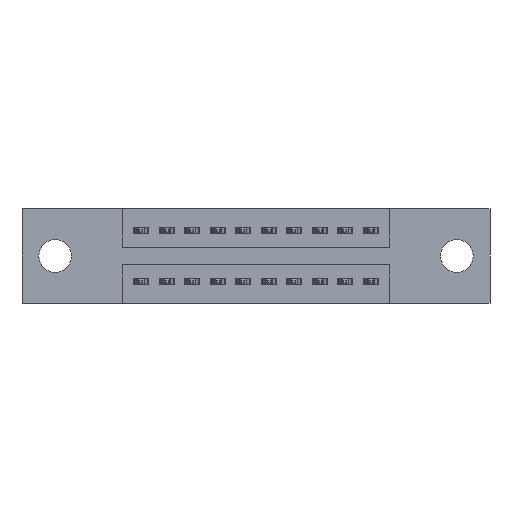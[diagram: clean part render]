
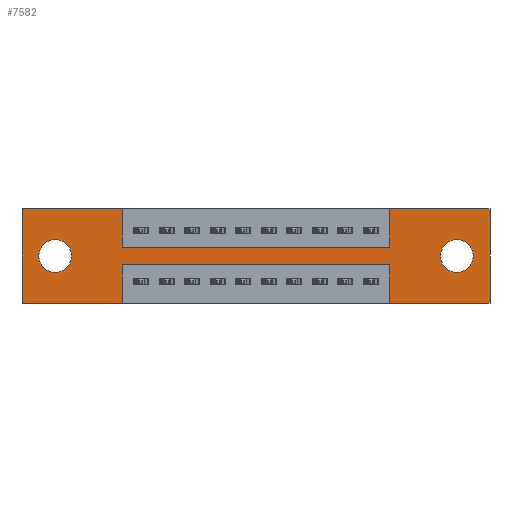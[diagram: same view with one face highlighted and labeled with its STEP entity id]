
A CAD part, front view. The second image highlights one B-rep face of the part: STEP entity #7582.
In plain terms, the highlighted planar face has unit normal (0, -1, 0).
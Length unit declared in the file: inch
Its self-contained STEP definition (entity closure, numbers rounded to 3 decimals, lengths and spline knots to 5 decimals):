
#117 = ORIENTED_EDGE ( 'NONE', *, *, #8578, .T. ) ;
#363 = DIRECTION ( 'NONE',  ( 0., 0., 1. ) ) ;
#426 = EDGE_CURVE ( 'NONE', #10131, #4651, #6226, .T. ) ;
#573 = CIRCLE ( 'NONE', #4026, 0.064 ) ;
#599 = EDGE_CURVE ( 'NONE', #11635, #8433, #9215, .T. ) ;
#674 = DIRECTION ( 'NONE',  ( 0., 1., 0. ) ) ;
#698 = ORIENTED_EDGE ( 'NONE', *, *, #4760, .T. ) ;
#797 = VERTEX_POINT ( 'NONE', #4921 ) ;
#798 = DIRECTION ( 'NONE',  ( 0., 1., 0. ) ) ;
#901 = CARTESIAN_POINT ( 'NONE',  ( 1.4425, 0., -0.15 ) ) ;
#910 = DIRECTION ( 'NONE',  ( -1., 0., 0. ) ) ;
#1157 = ORIENTED_EDGE ( 'NONE', *, *, #7552, .F. ) ;
#1232 = CARTESIAN_POINT ( 'NONE',  ( 1.705, 0., -0.185 ) ) ;
#1618 = CARTESIAN_POINT ( 'NONE',  ( 0.13, 0., -0.185 ) ) ;
#1696 = LINE ( 'NONE', #4581, #8347 ) ;
#1740 = CARTESIAN_POINT ( 'NONE',  ( 0.13, 0., -0.121 ) ) ;
#1905 = VERTEX_POINT ( 'NONE', #1740 ) ;
#2096 = LINE ( 'NONE', #7537, #6650 ) ;
#2200 = DIRECTION ( 'NONE',  ( 0., 1., 0. ) ) ;
#2248 = VECTOR ( 'NONE', #10464, 39.37008 ) ;
#2322 = CIRCLE ( 'NONE', #6504, 0.064 ) ;
#2341 = DIRECTION ( 'NONE',  ( 0., -1., 0. ) ) ;
#2364 = CARTESIAN_POINT ( 'NONE',  ( 1.4425, 0., 0. ) ) ;
#2391 = VECTOR ( 'NONE', #3422, 39.37008 ) ;
#2468 = VECTOR ( 'NONE', #910, 39.37008 ) ;
#2492 = CARTESIAN_POINT ( 'NONE',  ( 0., 0., 0. ) ) ;
#2693 = VECTOR ( 'NONE', #5225, 39.37008 ) ;
#2758 = CARTESIAN_POINT ( 'NONE',  ( 1.835, 0., 0. ) ) ;
#2976 = CARTESIAN_POINT ( 'NONE',  ( 0., 0., 0. ) ) ;
#2991 = CIRCLE ( 'NONE', #7882, 0.064 ) ;
#3112 = EDGE_CURVE ( 'NONE', #9132, #5000, #3172, .T. ) ;
#3153 = LINE ( 'NONE', #5531, #10993 ) ;
#3172 = LINE ( 'NONE', #9256, #10413 ) ;
#3190 = VERTEX_POINT ( 'NONE', #10410 ) ;
#3262 = CARTESIAN_POINT ( 'NONE',  ( 1.705, 0., -0.249 ) ) ;
#3422 = DIRECTION ( 'NONE',  ( 1., 0., 0. ) ) ;
#3828 = CARTESIAN_POINT ( 'NONE',  ( 1.4425, 0., -0.37 ) ) ;
#3977 = DIRECTION ( 'NONE',  ( 0., 0., -1. ) ) ;
#4008 = EDGE_LOOP ( 'NONE', ( #9153, #8576, #11238, #9944, #4397, #11677, #10538, #4881, #1157, #10408, #7628, #12001 ) ) ;
#4026 = AXIS2_PLACEMENT_3D ( 'NONE', #1618, #674, #10848 ) ;
#4397 = ORIENTED_EDGE ( 'NONE', *, *, #9378, .F. ) ;
#4581 = CARTESIAN_POINT ( 'NONE',  ( 0., 0., 0. ) ) ;
#4601 = CARTESIAN_POINT ( 'NONE',  ( 0., 0., -0.37 ) ) ;
#4606 = EDGE_CURVE ( 'NONE', #4651, #7779, #1696, .T. ) ;
#4651 = VERTEX_POINT ( 'NONE', #7466 ) ;
#4669 = EDGE_LOOP ( 'NONE', ( #698, #10073 ) ) ;
#4760 = EDGE_CURVE ( 'NONE', #797, #10524, #2991, .T. ) ;
#4812 = CARTESIAN_POINT ( 'NONE',  ( 0.3925, 0., 0. ) ) ;
#4881 = ORIENTED_EDGE ( 'NONE', *, *, #11899, .F. ) ;
#4921 = CARTESIAN_POINT ( 'NONE',  ( 1.705, 0., -0.121 ) ) ;
#5000 = VERTEX_POINT ( 'NONE', #2976 ) ;
#5011 = DIRECTION ( 'NONE',  ( 0., 1., 0. ) ) ;
#5141 = CARTESIAN_POINT ( 'NONE',  ( 0.13, 0., -0.185 ) ) ;
#5225 = DIRECTION ( 'NONE',  ( 0., 0., 1. ) ) ;
#5465 = AXIS2_PLACEMENT_3D ( 'NONE', #1232, #2200, #3977 ) ;
#5531 = CARTESIAN_POINT ( 'NONE',  ( 0.3925, 0., -0.37 ) ) ;
#5583 = CARTESIAN_POINT ( 'NONE',  ( 0., 0., -0.37 ) ) ;
#6120 = DIRECTION ( 'NONE',  ( 0., 0., -1. ) ) ;
#6155 = EDGE_CURVE ( 'NONE', #8433, #8966, #8026, .T. ) ;
#6226 = LINE ( 'NONE', #2364, #2693 ) ;
#6349 = EDGE_CURVE ( 'NONE', #8966, #8856, #9642, .T. ) ;
#6410 = DIRECTION ( 'NONE',  ( 0., 0., -1. ) ) ;
#6416 = EDGE_CURVE ( 'NONE', #5000, #10974, #8170, .T. ) ;
#6419 = LINE ( 'NONE', #2758, #10865 ) ;
#6421 = AXIS2_PLACEMENT_3D ( 'NONE', #9003, #2341, #6120 ) ;
#6456 = LINE ( 'NONE', #11444, #9891 ) ;
#6504 = AXIS2_PLACEMENT_3D ( 'NONE', #5141, #5011, #363 ) ;
#6565 = DIRECTION ( 'NONE',  ( 0., 0., -1. ) ) ;
#6650 = VECTOR ( 'NONE', #9454, 39.37008 ) ;
#6758 = FACE_BOUND ( 'NONE', #7322, .T. ) ;
#7044 = DIRECTION ( 'NONE',  ( -1., 0., 0. ) ) ;
#7322 = EDGE_LOOP ( 'NONE', ( #117, #10649 ) ) ;
#7332 = CIRCLE ( 'NONE', #5465, 0.064 ) ;
#7386 = DIRECTION ( 'NONE',  ( 1., 0., 0. ) ) ;
#7466 = CARTESIAN_POINT ( 'NONE',  ( 1.4425, 0., 0. ) ) ;
#7503 = VERTEX_POINT ( 'NONE', #10505 ) ;
#7531 = FACE_OUTER_BOUND ( 'NONE', #4008, .T. ) ;
#7537 = CARTESIAN_POINT ( 'NONE',  ( 0.3925, 0., -0.15 ) ) ;
#7552 = EDGE_CURVE ( 'NONE', #10974, #3190, #6456, .T. ) ;
#7582 = ADVANCED_FACE ( 'NONE', ( #11938, #6758, #7531 ), #8014, .T. ) ;
#7628 = ORIENTED_EDGE ( 'NONE', *, *, #3112, .F. ) ;
#7747 = CARTESIAN_POINT ( 'NONE',  ( 1.4425, 0., -0.37 ) ) ;
#7779 = VERTEX_POINT ( 'NONE', #10816 ) ;
#7882 = AXIS2_PLACEMENT_3D ( 'NONE', #8320, #798, #9336 ) ;
#7947 = CARTESIAN_POINT ( 'NONE',  ( 1.835, 0., -0.37 ) ) ;
#8014 = PLANE ( 'NONE',  #6421 ) ;
#8026 = LINE ( 'NONE', #3828, #2248 ) ;
#8170 = LINE ( 'NONE', #2492, #2391 ) ;
#8320 = CARTESIAN_POINT ( 'NONE',  ( 1.705, 0., -0.185 ) ) ;
#8347 = VECTOR ( 'NONE', #7386, 39.37008 ) ;
#8433 = VERTEX_POINT ( 'NONE', #7747 ) ;
#8576 = ORIENTED_EDGE ( 'NONE', *, *, #6349, .F. ) ;
#8578 = EDGE_CURVE ( 'NONE', #1905, #7503, #573, .T. ) ;
#8680 = EDGE_CURVE ( 'NONE', #10098, #9132, #10592, .T. ) ;
#8856 = VERTEX_POINT ( 'NONE', #10693 ) ;
#8966 = VERTEX_POINT ( 'NONE', #10539 ) ;
#9003 = CARTESIAN_POINT ( 'NONE',  ( 0., 0., -0.37 ) ) ;
#9132 = VERTEX_POINT ( 'NONE', #4601 ) ;
#9153 = ORIENTED_EDGE ( 'NONE', *, *, #10016, .F. ) ;
#9213 = EDGE_CURVE ( 'NONE', #7503, #1905, #2322, .T. ) ;
#9215 = LINE ( 'NONE', #5583, #9934 ) ;
#9256 = CARTESIAN_POINT ( 'NONE',  ( 0., 0., 0. ) ) ;
#9336 = DIRECTION ( 'NONE',  ( 0., 0., -1. ) ) ;
#9378 = EDGE_CURVE ( 'NONE', #7779, #11635, #6419, .T. ) ;
#9454 = DIRECTION ( 'NONE',  ( 1., 0., 0. ) ) ;
#9480 = DIRECTION ( 'NONE',  ( -1., 0., 0. ) ) ;
#9642 = LINE ( 'NONE', #11738, #11828 ) ;
#9800 = EDGE_CURVE ( 'NONE', #10524, #797, #7332, .T. ) ;
#9891 = VECTOR ( 'NONE', #6565, 39.37008 ) ;
#9934 = VECTOR ( 'NONE', #9480, 39.37008 ) ;
#9944 = ORIENTED_EDGE ( 'NONE', *, *, #599, .F. ) ;
#10016 = EDGE_CURVE ( 'NONE', #8856, #10098, #3153, .T. ) ;
#10073 = ORIENTED_EDGE ( 'NONE', *, *, #9800, .T. ) ;
#10098 = VERTEX_POINT ( 'NONE', #11120 ) ;
#10131 = VERTEX_POINT ( 'NONE', #901 ) ;
#10306 = CARTESIAN_POINT ( 'NONE',  ( 0., 0., -0.37 ) ) ;
#10408 = ORIENTED_EDGE ( 'NONE', *, *, #6416, .F. ) ;
#10410 = CARTESIAN_POINT ( 'NONE',  ( 0.3925, 0., -0.15 ) ) ;
#10413 = VECTOR ( 'NONE', #11158, 39.37008 ) ;
#10464 = DIRECTION ( 'NONE',  ( 0., 0., 1. ) ) ;
#10505 = CARTESIAN_POINT ( 'NONE',  ( 0.13, 0., -0.249 ) ) ;
#10524 = VERTEX_POINT ( 'NONE', #3262 ) ;
#10538 = ORIENTED_EDGE ( 'NONE', *, *, #426, .F. ) ;
#10539 = CARTESIAN_POINT ( 'NONE',  ( 1.4425, 0., -0.22 ) ) ;
#10592 = LINE ( 'NONE', #10306, #2468 ) ;
#10649 = ORIENTED_EDGE ( 'NONE', *, *, #9213, .T. ) ;
#10693 = CARTESIAN_POINT ( 'NONE',  ( 0.3925, 0., -0.22 ) ) ;
#10816 = CARTESIAN_POINT ( 'NONE',  ( 1.835, 0., 0. ) ) ;
#10848 = DIRECTION ( 'NONE',  ( 0., 0., 1. ) ) ;
#10865 = VECTOR ( 'NONE', #11293, 39.37008 ) ;
#10974 = VERTEX_POINT ( 'NONE', #4812 ) ;
#10993 = VECTOR ( 'NONE', #6410, 39.37008 ) ;
#11120 = CARTESIAN_POINT ( 'NONE',  ( 0.3925, 0., -0.37 ) ) ;
#11158 = DIRECTION ( 'NONE',  ( 0., 0., 1. ) ) ;
#11238 = ORIENTED_EDGE ( 'NONE', *, *, #6155, .F. ) ;
#11293 = DIRECTION ( 'NONE',  ( 0., 0., -1. ) ) ;
#11444 = CARTESIAN_POINT ( 'NONE',  ( 0.3925, 0., 0. ) ) ;
#11635 = VERTEX_POINT ( 'NONE', #7947 ) ;
#11677 = ORIENTED_EDGE ( 'NONE', *, *, #4606, .F. ) ;
#11738 = CARTESIAN_POINT ( 'NONE',  ( 0.3925, 0., -0.22 ) ) ;
#11828 = VECTOR ( 'NONE', #7044, 39.37008 ) ;
#11899 = EDGE_CURVE ( 'NONE', #3190, #10131, #2096, .T. ) ;
#11938 = FACE_BOUND ( 'NONE', #4669, .T. ) ;
#12001 = ORIENTED_EDGE ( 'NONE', *, *, #8680, .F. ) ;
